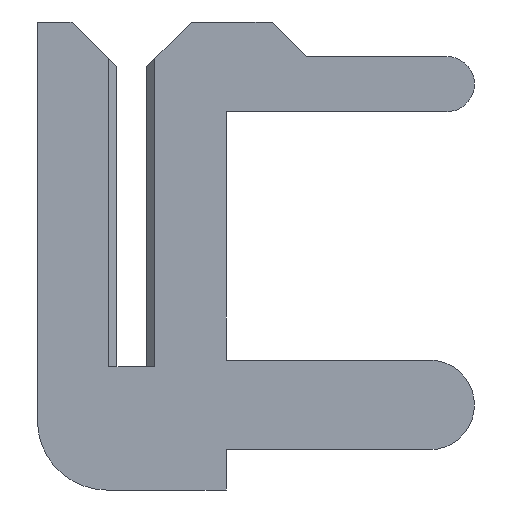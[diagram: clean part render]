
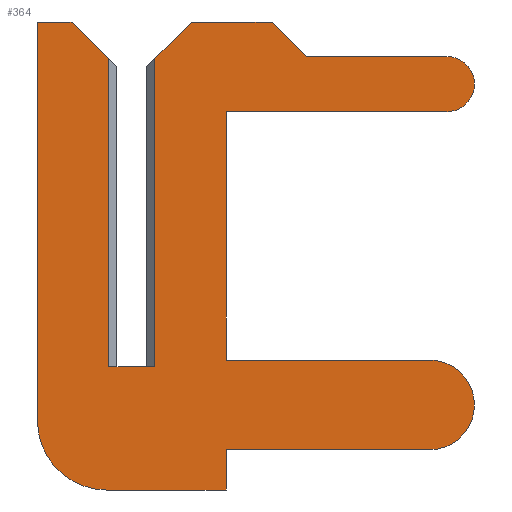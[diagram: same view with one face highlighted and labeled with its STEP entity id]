
A CAD part, left-side view. The second image highlights one B-rep face of the part: STEP entity #364.
In plain terms, the highlighted planar face has unit normal (-1, 0, 0).
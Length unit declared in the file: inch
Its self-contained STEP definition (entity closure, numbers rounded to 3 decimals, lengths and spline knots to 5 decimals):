
#3 = CARTESIAN_POINT ( 'NONE',  ( -0.01, 0.011, -0.0235 ) ) ;
#6 = CARTESIAN_POINT ( 'NONE',  ( -0.01, 0.041, 0.15 ) ) ;
#9 = ORIENTED_EDGE ( 'NONE', *, *, #514, .F. ) ;
#10 = VECTOR ( 'NONE', #161, 39.37008 ) ;
#31 = EDGE_CURVE ( 'NONE', #678, #671, #241, .T. ) ;
#34 = VECTOR ( 'NONE', #778, 39.37008 ) ;
#35 = ORIENTED_EDGE ( 'NONE', *, *, #1090, .F. ) ;
#46 = CARTESIAN_POINT ( 'NONE',  ( -0.01, 0.01, -0.0235 ) ) ;
#48 = CARTESIAN_POINT ( 'NONE',  ( -0.01, -0.041, 0.003 ) ) ;
#59 = CARTESIAN_POINT ( 'NONE',  ( -0.01, -0.076, 0.135 ) ) ;
#61 = EDGE_CURVE ( 'NONE', #313, #794, #887, .T. ) ;
#82 = CARTESIAN_POINT ( 'NONE',  ( -0.01, 0.041, -0.0235 ) ) ;
#86 = CARTESIAN_POINT ( 'NONE',  ( -0.01, 0.011, -0.0535 ) ) ;
#88 = VECTOR ( 'NONE', #563, 39.37008 ) ;
#90 = VERTEX_POINT ( 'NONE', #322 ) ;
#92 = VECTOR ( 'NONE', #504, 39.37008 ) ;
#102 = EDGE_CURVE ( 'NONE', #678, #358, #919, .T. ) ;
#108 = VECTOR ( 'NONE', #369, 39.37008 ) ;
#119 = LINE ( 'NONE', #941, #166 ) ;
#140 = EDGE_LOOP ( 'NONE', ( #1060, #1021, #920, #325, #792, #386, #155, #697, #9, #1094, #1038, #551, #799, #1072, #830, #35, #925, #895, #468 ) ) ;
#141 = CARTESIAN_POINT ( 'NONE',  ( -0.01, 0.01, 0. ) ) ;
#142 = EDGE_CURVE ( 'NONE', #815, #712, #486, .T. ) ;
#147 = CARTESIAN_POINT ( 'NONE',  ( -0.01, 0.026, 0.15 ) ) ;
#149 = CIRCLE ( 'NONE', #593, 0.0195 ) ;
#150 = CARTESIAN_POINT ( 'NONE',  ( -0.01, -0.1295, -0.036 ) ) ;
#155 = ORIENTED_EDGE ( 'NONE', *, *, #1065, .F. ) ;
#159 = DIRECTION ( 'NONE',  ( 1., 0., 0. ) ) ;
#161 = DIRECTION ( 'NONE',  ( 0., -0.707, -0.707 ) ) ;
#166 = VECTOR ( 'NONE', #1024, 39.37008 ) ;
#180 = DIRECTION ( 'NONE',  ( -1., 0., 0. ) ) ;
#185 = VECTOR ( 'NONE', #736, 39.37008 ) ;
#188 = VERTEX_POINT ( 'NONE', #406 ) ;
#190 = CARTESIAN_POINT ( 'NONE',  ( -0.01, -0.0065, 0.1305 ) ) ;
#192 = CARTESIAN_POINT ( 'NONE',  ( -0.01, 0.0065, 0.1305 ) ) ;
#200 = LINE ( 'NONE', #432, #1057 ) ;
#209 = EDGE_CURVE ( 'NONE', #712, #188, #1042, .T. ) ;
#211 = VECTOR ( 'NONE', #742, 39.37008 ) ;
#213 = VECTOR ( 'NONE', #645, 39.37008 ) ;
#223 = VERTEX_POINT ( 'NONE', #82 ) ;
#228 = VERTEX_POINT ( 'NONE', #86 ) ;
#237 = EDGE_CURVE ( 'NONE', #590, #90, #200, .T. ) ;
#241 = LINE ( 'NONE', #46, #213 ) ;
#244 = CARTESIAN_POINT ( 'NONE',  ( -0.01, 0.026, 0.15 ) ) ;
#245 = CARTESIAN_POINT ( 'NONE',  ( -0.01, 0.0065, 0. ) ) ;
#256 = DIRECTION ( 'NONE',  ( 0., 0., 1. ) ) ;
#260 = DIRECTION ( 'NONE',  ( 0., -1., 0. ) ) ;
#267 = VECTOR ( 'NONE', #443, 39.37008 ) ;
#313 = VERTEX_POINT ( 'NONE', #1003 ) ;
#319 = CARTESIAN_POINT ( 'NONE',  ( -0.01, -0.041, -0.036 ) ) ;
#322 = CARTESIAN_POINT ( 'NONE',  ( -0.01, -0.1295, 0.003 ) ) ;
#325 = ORIENTED_EDGE ( 'NONE', *, *, #31, .T. ) ;
#341 = CARTESIAN_POINT ( 'NONE',  ( -0.01, -0.026, 0.15 ) ) ;
#342 = LINE ( 'NONE', #190, #34 ) ;
#346 = LINE ( 'NONE', #192, #108 ) ;
#356 = LINE ( 'NONE', #865, #589 ) ;
#358 = VERTEX_POINT ( 'NONE', #850 ) ;
#364 = ADVANCED_FACE ( 'NONE', ( #1006 ), #517, .T. ) ;
#369 = DIRECTION ( 'NONE',  ( 0., -0.707, -0.707 ) ) ;
#373 = EDGE_CURVE ( 'NONE', #228, #223, #525, .T. ) ;
#376 = VERTEX_POINT ( 'NONE', #1015 ) ;
#386 = ORIENTED_EDGE ( 'NONE', *, *, #938, .F. ) ;
#397 = EDGE_CURVE ( 'NONE', #889, #671, #346, .T. ) ;
#399 = DIRECTION ( 'NONE',  ( 0., 1., 0. ) ) ;
#404 = CARTESIAN_POINT ( 'NONE',  ( -0.01, -0.01, 0.15 ) ) ;
#406 = CARTESIAN_POINT ( 'NONE',  ( -0.01, -0.041, -0.0535 ) ) ;
#411 = CARTESIAN_POINT ( 'NONE',  ( -0.01, -0.076, 0.135 ) ) ;
#412 = VERTEX_POINT ( 'NONE', #6 ) ;
#413 = VERTEX_POINT ( 'NONE', #696 ) ;
#421 = CARTESIAN_POINT ( 'NONE',  ( -0.01, -0.041, -0.036 ) ) ;
#430 = CARTESIAN_POINT ( 'NONE',  ( -0.01, -0.137, 0.123 ) ) ;
#432 = CARTESIAN_POINT ( 'NONE',  ( -0.01, -0.1295, 0.003 ) ) ;
#434 = CARTESIAN_POINT ( 'NONE',  ( -0.01, -0.041, -0.0535 ) ) ;
#443 = DIRECTION ( 'NONE',  ( 0., 0., -1. ) ) ;
#446 = DIRECTION ( 'NONE',  ( 0., 0., 1. ) ) ;
#452 = LINE ( 'NONE', #1052, #88 ) ;
#467 = LINE ( 'NONE', #244, #211 ) ;
#468 = ORIENTED_EDGE ( 'NONE', *, *, #901, .F. ) ;
#476 = EDGE_CURVE ( 'NONE', #790, #1022, #342, .T. ) ;
#486 = LINE ( 'NONE', #421, #92 ) ;
#504 = DIRECTION ( 'NONE',  ( 0., 1., 0. ) ) ;
#514 = EDGE_CURVE ( 'NONE', #188, #228, #119, .T. ) ;
#515 = DIRECTION ( 'NONE',  ( 1., 0., 0. ) ) ;
#517 = PLANE ( 'NONE',  #576 ) ;
#525 = CIRCLE ( 'NONE', #641, 0.03 ) ;
#537 = EDGE_CURVE ( 'NONE', #413, #376, #356, .T. ) ;
#548 = EDGE_CURVE ( 'NONE', #376, #590, #452, .T. ) ;
#551 = ORIENTED_EDGE ( 'NONE', *, *, #930, .F. ) ;
#555 = DIRECTION ( 'NONE',  ( 0., -1., 0. ) ) ;
#561 = EDGE_CURVE ( 'NONE', #794, #577, #992, .T. ) ;
#563 = DIRECTION ( 'NONE',  ( 0., 0., -1. ) ) ;
#568 = CARTESIAN_POINT ( 'NONE',  ( -0.01, -0.01, 0.134 ) ) ;
#576 = AXIS2_PLACEMENT_3D ( 'NONE', #1093, #180, #765 ) ;
#577 = VERTEX_POINT ( 'NONE', #726 ) ;
#582 = DIRECTION ( 'NONE',  ( 0., -1., 0. ) ) ;
#589 = VECTOR ( 'NONE', #399, 39.37008 ) ;
#590 = VERTEX_POINT ( 'NONE', #48 ) ;
#593 = AXIS2_PLACEMENT_3D ( 'NONE', #1076, #159, #256 ) ;
#616 = LINE ( 'NONE', #404, #635 ) ;
#622 = DIRECTION ( 'NONE',  ( 1., 0., 0. ) ) ;
#623 = EDGE_CURVE ( 'NONE', #790, #358, #616, .T. ) ;
#635 = VECTOR ( 'NONE', #1062, 39.37008 ) ;
#641 = AXIS2_PLACEMENT_3D ( 'NONE', #3, #622, #446 ) ;
#645 = DIRECTION ( 'NONE',  ( 0., 0., 1. ) ) ;
#647 = LINE ( 'NONE', #751, #185 ) ;
#671 = VERTEX_POINT ( 'NONE', #890 ) ;
#678 = VERTEX_POINT ( 'NONE', #141 ) ;
#681 = DIRECTION ( 'NONE',  ( 0., 0., 1. ) ) ;
#696 = CARTESIAN_POINT ( 'NONE',  ( -0.01, -0.137, 0.111 ) ) ;
#697 = ORIENTED_EDGE ( 'NONE', *, *, #373, .F. ) ;
#712 = VERTEX_POINT ( 'NONE', #319 ) ;
#723 = CARTESIAN_POINT ( 'NONE',  ( -0.01, -0.137, 0.135 ) ) ;
#726 = CARTESIAN_POINT ( 'NONE',  ( -0.01, -0.137, 0.135 ) ) ;
#736 = DIRECTION ( 'NONE',  ( 0., -1., 0. ) ) ;
#737 = AXIS2_PLACEMENT_3D ( 'NONE', #430, #515, #681 ) ;
#742 = DIRECTION ( 'NONE',  ( 0., -1., 0. ) ) ;
#751 = CARTESIAN_POINT ( 'NONE',  ( -0.01, -0.026, 0.15 ) ) ;
#765 = DIRECTION ( 'NONE',  ( 0., 0., 1. ) ) ;
#778 = DIRECTION ( 'NONE',  ( 0., -0.707, 0.707 ) ) ;
#790 = VERTEX_POINT ( 'NONE', #568 ) ;
#792 = ORIENTED_EDGE ( 'NONE', *, *, #397, .F. ) ;
#794 = VERTEX_POINT ( 'NONE', #59 ) ;
#799 = ORIENTED_EDGE ( 'NONE', *, *, #237, .F. ) ;
#815 = VERTEX_POINT ( 'NONE', #150 ) ;
#830 = ORIENTED_EDGE ( 'NONE', *, *, #537, .F. ) ;
#849 = DIRECTION ( 'NONE',  ( 0., 0., 1. ) ) ;
#850 = CARTESIAN_POINT ( 'NONE',  ( -0.01, -0.01, 0. ) ) ;
#857 = LINE ( 'NONE', #931, #955 ) ;
#865 = CARTESIAN_POINT ( 'NONE',  ( -0.01, -0.041, 0.111 ) ) ;
#887 = LINE ( 'NONE', #411, #10 ) ;
#889 = VERTEX_POINT ( 'NONE', #147 ) ;
#890 = CARTESIAN_POINT ( 'NONE',  ( -0.01, 0.01, 0.134 ) ) ;
#895 = ORIENTED_EDGE ( 'NONE', *, *, #61, .F. ) ;
#901 = EDGE_CURVE ( 'NONE', #1022, #313, #647, .T. ) ;
#903 = CIRCLE ( 'NONE', #737, 0.012 ) ;
#919 = LINE ( 'NONE', #245, #979 ) ;
#920 = ORIENTED_EDGE ( 'NONE', *, *, #102, .F. ) ;
#925 = ORIENTED_EDGE ( 'NONE', *, *, #561, .F. ) ;
#930 = EDGE_CURVE ( 'NONE', #90, #815, #149, .T. ) ;
#931 = CARTESIAN_POINT ( 'NONE',  ( -0.01, 0.041, 0.15 ) ) ;
#938 = EDGE_CURVE ( 'NONE', #412, #889, #467, .T. ) ;
#941 = CARTESIAN_POINT ( 'NONE',  ( -0.01, 0.011, -0.0535 ) ) ;
#955 = VECTOR ( 'NONE', #849, 39.37008 ) ;
#976 = VECTOR ( 'NONE', #555, 39.37008 ) ;
#979 = VECTOR ( 'NONE', #582, 39.37008 ) ;
#992 = LINE ( 'NONE', #723, #976 ) ;
#1003 = CARTESIAN_POINT ( 'NONE',  ( -0.01, -0.061, 0.15 ) ) ;
#1006 = FACE_OUTER_BOUND ( 'NONE', #140, .T. ) ;
#1015 = CARTESIAN_POINT ( 'NONE',  ( -0.01, -0.041, 0.111 ) ) ;
#1021 = ORIENTED_EDGE ( 'NONE', *, *, #623, .T. ) ;
#1022 = VERTEX_POINT ( 'NONE', #341 ) ;
#1024 = DIRECTION ( 'NONE',  ( 0., 1., 0. ) ) ;
#1038 = ORIENTED_EDGE ( 'NONE', *, *, #142, .F. ) ;
#1042 = LINE ( 'NONE', #434, #267 ) ;
#1052 = CARTESIAN_POINT ( 'NONE',  ( -0.01, -0.041, 0.003 ) ) ;
#1057 = VECTOR ( 'NONE', #260, 39.37008 ) ;
#1060 = ORIENTED_EDGE ( 'NONE', *, *, #476, .F. ) ;
#1062 = DIRECTION ( 'NONE',  ( 0., 0., -1. ) ) ;
#1065 = EDGE_CURVE ( 'NONE', #223, #412, #857, .T. ) ;
#1072 = ORIENTED_EDGE ( 'NONE', *, *, #548, .F. ) ;
#1076 = CARTESIAN_POINT ( 'NONE',  ( -0.01, -0.1295, -0.0165 ) ) ;
#1090 = EDGE_CURVE ( 'NONE', #577, #413, #903, .T. ) ;
#1093 = CARTESIAN_POINT ( 'NONE',  ( -0.01, 0.011, -0.0235 ) ) ;
#1094 = ORIENTED_EDGE ( 'NONE', *, *, #209, .F. ) ;
